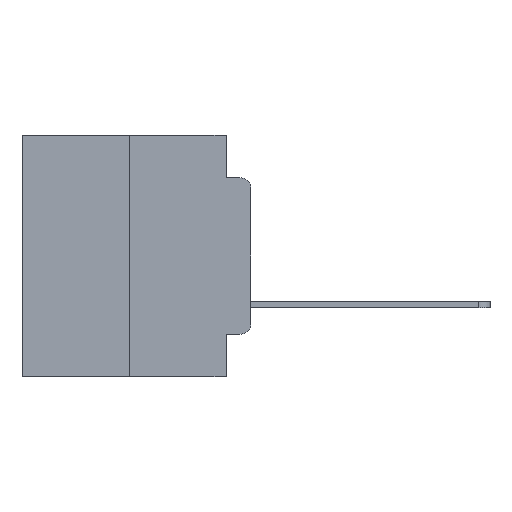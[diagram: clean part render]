
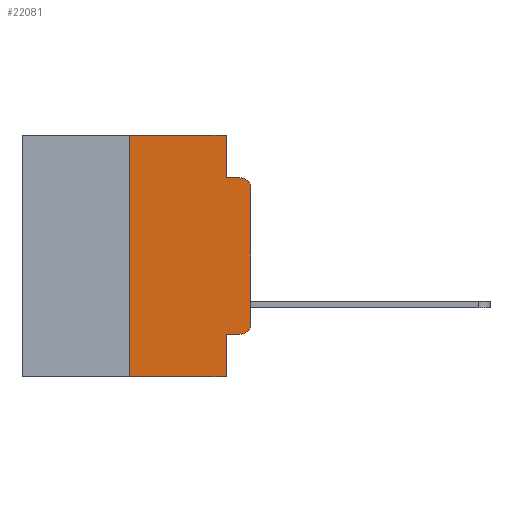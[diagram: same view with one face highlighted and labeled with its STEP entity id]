
A CAD part, left-side view. The second image highlights one B-rep face of the part: STEP entity #22081.
In plain terms, the highlighted planar face has unit normal (-1, 0, 0).
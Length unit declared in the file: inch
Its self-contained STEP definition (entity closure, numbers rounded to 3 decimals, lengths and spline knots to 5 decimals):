
#521 = LINE ( 'NONE', #21696, #21871 ) ;
#1053 = VECTOR ( 'NONE', #9738, 39.37008 ) ;
#1336 = DIRECTION ( 'NONE',  ( 0., 0., -1. ) ) ;
#1601 = DIRECTION ( 'NONE',  ( 1., 0., 0. ) ) ;
#2134 = AXIS2_PLACEMENT_3D ( 'NONE', #20358, #26886, #22399 ) ;
#2208 = VECTOR ( 'NONE', #18747, 39.37008 ) ;
#2513 = VERTEX_POINT ( 'NONE', #17272 ) ;
#2570 = CARTESIAN_POINT ( 'NONE',  ( 0., 0.02, -0.0885 ) ) ;
#3067 = CARTESIAN_POINT ( 'NONE',  ( 0., 0.051, -0.4115 ) ) ;
#3591 = CARTESIAN_POINT ( 'NONE',  ( 0., 0.473, 0. ) ) ;
#3693 = VERTEX_POINT ( 'NONE', #18286 ) ;
#3718 = ORIENTED_EDGE ( 'NONE', *, *, #6334, .F. ) ;
#3990 = VERTEX_POINT ( 'NONE', #12895 ) ;
#4671 = VECTOR ( 'NONE', #19895, 39.37008 ) ;
#6334 = EDGE_CURVE ( 'NONE', #3693, #12194, #521, .T. ) ;
#6404 = VERTEX_POINT ( 'NONE', #9398 ) ;
#7156 = LINE ( 'NONE', #25548, #21089 ) ;
#7406 = CARTESIAN_POINT ( 'NONE',  ( 0., 0., 0. ) ) ;
#7558 = CARTESIAN_POINT ( 'NONE',  ( 0., 0.051, -0.0885 ) ) ;
#8387 = VECTOR ( 'NONE', #16744, 39.37008 ) ;
#8581 = CARTESIAN_POINT ( 'NONE',  ( 0., 0.25, 0. ) ) ;
#8582 = LINE ( 'NONE', #16847, #2208 ) ;
#9398 = CARTESIAN_POINT ( 'NONE',  ( 0., 0.25, 0. ) ) ;
#9738 = DIRECTION ( 'NONE',  ( 0., -1., 0. ) ) ;
#9932 = VECTOR ( 'NONE', #17797, 39.37008 ) ;
#10235 = ORIENTED_EDGE ( 'NONE', *, *, #24787, .F. ) ;
#10629 = CARTESIAN_POINT ( 'NONE',  ( 0., 0.051, -0.0885 ) ) ;
#11182 = DIRECTION ( 'NONE',  ( -1., 0., 0. ) ) ;
#11884 = ORIENTED_EDGE ( 'NONE', *, *, #17656, .T. ) ;
#12194 = VERTEX_POINT ( 'NONE', #10629 ) ;
#12449 = EDGE_LOOP ( 'NONE', ( #17699, #27033, #20013, #3718, #16042, #10235, #20589, #19191, #17689, #11884 ) ) ;
#12895 = CARTESIAN_POINT ( 'NONE',  ( 0., 0.25, -0.5 ) ) ;
#12954 = DIRECTION ( 'NONE',  ( 0., 0., 1. ) ) ;
#12959 = DIRECTION ( 'NONE',  ( 0., 0., -1. ) ) ;
#12983 = CIRCLE ( 'NONE', #2134, 0.02 ) ;
#13400 = VERTEX_POINT ( 'NONE', #21270 ) ;
#13440 = VERTEX_POINT ( 'NONE', #19547 ) ;
#13695 = VERTEX_POINT ( 'NONE', #3067 ) ;
#14504 = EDGE_CURVE ( 'NONE', #24778, #24886, #12983, .T. ) ;
#14929 = LINE ( 'NONE', #7406, #9932 ) ;
#15116 = DIRECTION ( 'NONE',  ( 0., -1., 0. ) ) ;
#16042 = ORIENTED_EDGE ( 'NONE', *, *, #22558, .F. ) ;
#16094 = CARTESIAN_POINT ( 'NONE',  ( 0., 0.051, 0. ) ) ;
#16744 = DIRECTION ( 'NONE',  ( 0., -1., 0. ) ) ;
#16847 = CARTESIAN_POINT ( 'NONE',  ( 0., 0.473, -0.5 ) ) ;
#17272 = CARTESIAN_POINT ( 'NONE',  ( 0., 0.051, -0.5 ) ) ;
#17289 = CARTESIAN_POINT ( 'NONE',  ( 0., 0.02, -0.3915 ) ) ;
#17477 = DIRECTION ( 'NONE',  ( 0., 0., -1. ) ) ;
#17656 = EDGE_CURVE ( 'NONE', #13440, #13400, #17716, .T. ) ;
#17689 = ORIENTED_EDGE ( 'NONE', *, *, #25903, .T. ) ;
#17699 = ORIENTED_EDGE ( 'NONE', *, *, #25540, .T. ) ;
#17716 = CIRCLE ( 'NONE', #27582, 0.02 ) ;
#17797 = DIRECTION ( 'NONE',  ( 0., 0., 1. ) ) ;
#18286 = CARTESIAN_POINT ( 'NONE',  ( 0., 0.051, 0. ) ) ;
#18747 = DIRECTION ( 'NONE',  ( 0., -1., 0. ) ) ;
#19164 = CARTESIAN_POINT ( 'NONE',  ( 0., 0., -0.1085 ) ) ;
#19191 = ORIENTED_EDGE ( 'NONE', *, *, #26808, .F. ) ;
#19547 = CARTESIAN_POINT ( 'NONE',  ( 0., 0.02, -0.4115 ) ) ;
#19753 = EDGE_CURVE ( 'NONE', #3990, #2513, #8582, .T. ) ;
#19895 = DIRECTION ( 'NONE',  ( 0., 0., -1. ) ) ;
#20013 = ORIENTED_EDGE ( 'NONE', *, *, #26329, .F. ) ;
#20282 = VECTOR ( 'NONE', #12954, 39.37008 ) ;
#20358 = CARTESIAN_POINT ( 'NONE',  ( 0., 0.02, -0.1085 ) ) ;
#20589 = ORIENTED_EDGE ( 'NONE', *, *, #19753, .T. ) ;
#21089 = VECTOR ( 'NONE', #15116, 39.37008 ) ;
#21270 = CARTESIAN_POINT ( 'NONE',  ( 0., 0., -0.3915 ) ) ;
#21562 = AXIS2_PLACEMENT_3D ( 'NONE', #3591, #1601, #1336 ) ;
#21696 = CARTESIAN_POINT ( 'NONE',  ( 0., 0.051, 0. ) ) ;
#21871 = VECTOR ( 'NONE', #17477, 39.37008 ) ;
#22081 = ADVANCED_FACE ( 'NONE', ( #26447 ), #24809, .F. ) ;
#22399 = DIRECTION ( 'NONE',  ( 0., 0., -1. ) ) ;
#22558 = EDGE_CURVE ( 'NONE', #6404, #3693, #25093, .T. ) ;
#24496 = CARTESIAN_POINT ( 'NONE',  ( 0., 0.473, 0. ) ) ;
#24778 = VERTEX_POINT ( 'NONE', #19164 ) ;
#24787 = EDGE_CURVE ( 'NONE', #3990, #6404, #25964, .T. ) ;
#24809 = PLANE ( 'NONE',  #21562 ) ;
#24886 = VERTEX_POINT ( 'NONE', #2570 ) ;
#25093 = LINE ( 'NONE', #24496, #1053 ) ;
#25540 = EDGE_CURVE ( 'NONE', #13400, #24778, #14929, .T. ) ;
#25548 = CARTESIAN_POINT ( 'NONE',  ( 0., 0.051, -0.4115 ) ) ;
#25903 = EDGE_CURVE ( 'NONE', #13695, #13440, #7156, .T. ) ;
#25964 = LINE ( 'NONE', #8581, #20282 ) ;
#25994 = LINE ( 'NONE', #16094, #4671 ) ;
#26329 = EDGE_CURVE ( 'NONE', #12194, #24886, #27023, .T. ) ;
#26447 = FACE_OUTER_BOUND ( 'NONE', #12449, .T. ) ;
#26808 = EDGE_CURVE ( 'NONE', #13695, #2513, #25994, .T. ) ;
#26886 = DIRECTION ( 'NONE',  ( -1., 0., 0. ) ) ;
#27023 = LINE ( 'NONE', #7558, #8387 ) ;
#27033 = ORIENTED_EDGE ( 'NONE', *, *, #14504, .T. ) ;
#27582 = AXIS2_PLACEMENT_3D ( 'NONE', #17289, #11182, #12959 ) ;
